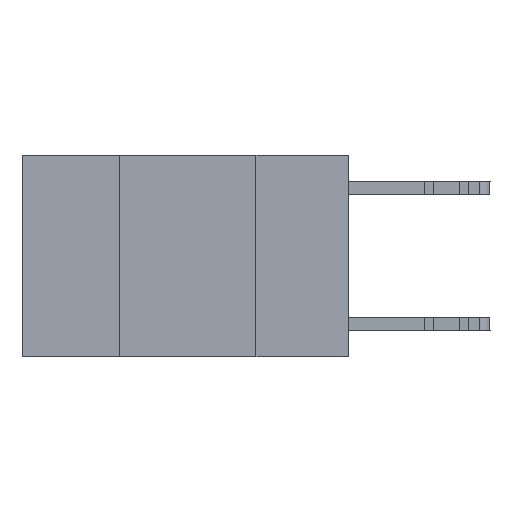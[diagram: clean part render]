
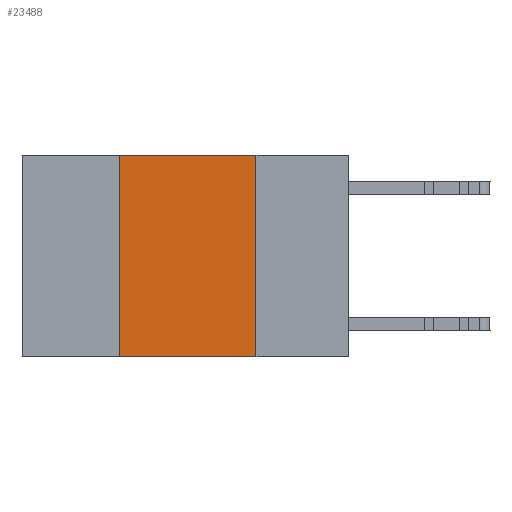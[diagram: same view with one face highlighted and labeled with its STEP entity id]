
A CAD part, left-side view. The second image highlights one B-rep face of the part: STEP entity #23488.
In plain terms, the highlighted planar face has unit normal (-1, 0, 0).
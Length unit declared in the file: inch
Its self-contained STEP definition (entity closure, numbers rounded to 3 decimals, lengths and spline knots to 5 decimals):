
#103 = CARTESIAN_POINT ( 'NONE',  ( 0., 0.42, 0. ) ) ;
#194 = ORIENTED_EDGE ( 'NONE', *, *, #5481, .F. ) ;
#1246 = CARTESIAN_POINT ( 'NONE',  ( 0., 0.6, 0. ) ) ;
#1815 = CARTESIAN_POINT ( 'NONE',  ( 0., 0.42, 0. ) ) ;
#2200 = CARTESIAN_POINT ( 'NONE',  ( 0., 0.17, 0. ) ) ;
#3170 = CARTESIAN_POINT ( 'NONE',  ( 0., 0.6, -0.37 ) ) ;
#3238 = DIRECTION ( 'NONE',  ( 1., 0., 0. ) ) ;
#3968 = VERTEX_POINT ( 'NONE', #18017 ) ;
#4637 = VERTEX_POINT ( 'NONE', #5119 ) ;
#5119 = CARTESIAN_POINT ( 'NONE',  ( 0., 0.42, -0.37 ) ) ;
#5342 = PLANE ( 'NONE',  #26547 ) ;
#5421 = EDGE_CURVE ( 'NONE', #4637, #6270, #18499, .T. ) ;
#5481 = EDGE_CURVE ( 'NONE', #13286, #3968, #13527, .T. ) ;
#6270 = VERTEX_POINT ( 'NONE', #1815 ) ;
#7588 = CARTESIAN_POINT ( 'NONE',  ( 0., 0.6, 0. ) ) ;
#8127 = EDGE_CURVE ( 'NONE', #6270, #13286, #17558, .T. ) ;
#8568 = VECTOR ( 'NONE', #13882, 39.37008 ) ;
#8945 = CARTESIAN_POINT ( 'NONE',  ( 0., 0.17, 0. ) ) ;
#9983 = DIRECTION ( 'NONE',  ( 0., 0., -1. ) ) ;
#10523 = DIRECTION ( 'NONE',  ( 0., -1., 0. ) ) ;
#11240 = ORIENTED_EDGE ( 'NONE', *, *, #8127, .F. ) ;
#12008 = ORIENTED_EDGE ( 'NONE', *, *, #5421, .F. ) ;
#12302 = LINE ( 'NONE', #3170, #20198 ) ;
#13286 = VERTEX_POINT ( 'NONE', #8945 ) ;
#13527 = LINE ( 'NONE', #2200, #20488 ) ;
#13882 = DIRECTION ( 'NONE',  ( 0., 0., 1. ) ) ;
#17343 = ORIENTED_EDGE ( 'NONE', *, *, #19113, .T. ) ;
#17558 = LINE ( 'NONE', #1246, #19305 ) ;
#18017 = CARTESIAN_POINT ( 'NONE',  ( 0., 0.17, -0.37 ) ) ;
#18209 = DIRECTION ( 'NONE',  ( 0., 0., -1. ) ) ;
#18499 = LINE ( 'NONE', #103, #8568 ) ;
#19113 = EDGE_CURVE ( 'NONE', #4637, #3968, #12302, .T. ) ;
#19305 = VECTOR ( 'NONE', #10523, 39.37008 ) ;
#20198 = VECTOR ( 'NONE', #28245, 39.37008 ) ;
#20488 = VECTOR ( 'NONE', #18209, 39.37008 ) ;
#21317 = FACE_OUTER_BOUND ( 'NONE', #25824, .T. ) ;
#23488 = ADVANCED_FACE ( 'NONE', ( #21317 ), #5342, .F. ) ;
#25824 = EDGE_LOOP ( 'NONE', ( #194, #11240, #12008, #17343 ) ) ;
#26547 = AXIS2_PLACEMENT_3D ( 'NONE', #7588, #3238, #9983 ) ;
#28245 = DIRECTION ( 'NONE',  ( 0., -1., 0. ) ) ;
